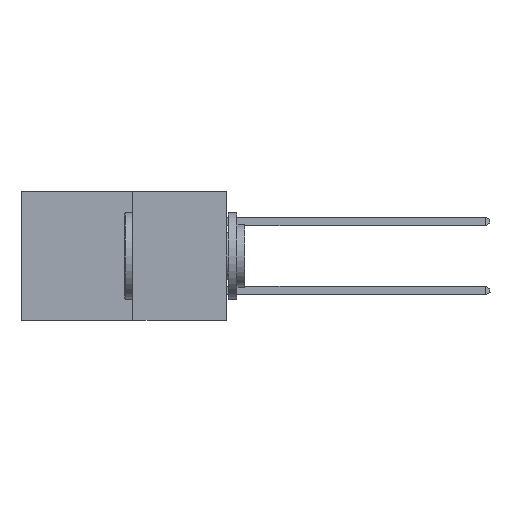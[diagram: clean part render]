
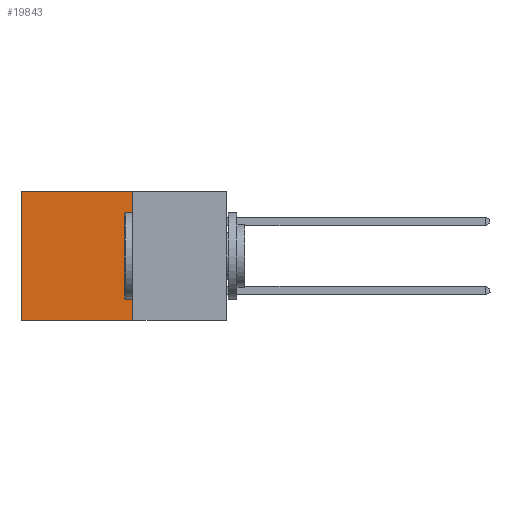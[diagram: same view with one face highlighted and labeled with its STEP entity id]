
A CAD part, left-side view. The second image highlights one B-rep face of the part: STEP entity #19843.
In plain terms, the highlighted planar face has unit normal (-1, 0, 0).
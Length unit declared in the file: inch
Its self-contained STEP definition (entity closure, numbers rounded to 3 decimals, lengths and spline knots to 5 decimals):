
#529 = EDGE_CURVE ( 'NONE', #17937, #8803, #17477, .T. ) ;
#590 = EDGE_CURVE ( 'NONE', #17795, #11460, #8284, .T. ) ;
#1274 = CARTESIAN_POINT ( 'NONE',  ( 0.277, 0.27, -0.37 ) ) ;
#2105 = CARTESIAN_POINT ( 'NONE',  ( 0.277, 0.27, 0. ) ) ;
#2142 = ORIENTED_EDGE ( 'NONE', *, *, #19636, .F. ) ;
#2510 = DIRECTION ( 'NONE',  ( 0., 0., -1. ) ) ;
#3514 = CARTESIAN_POINT ( 'NONE',  ( 0.277, 0.59, -0.37 ) ) ;
#4273 = EDGE_LOOP ( 'NONE', ( #13046, #2142, #16740, #10080 ) ) ;
#4469 = VECTOR ( 'NONE', #13166, 39.37008 ) ;
#4777 = CARTESIAN_POINT ( 'NONE',  ( 0.277, 0.59, -0.37 ) ) ;
#4942 = PLANE ( 'NONE',  #17885 ) ;
#6446 = CARTESIAN_POINT ( 'NONE',  ( 0.277, 0.27, 0. ) ) ;
#6563 = DIRECTION ( 'NONE',  ( 1., 0., 0. ) ) ;
#6834 = LINE ( 'NONE', #2105, #18254 ) ;
#7881 = LINE ( 'NONE', #1274, #12066 ) ;
#8284 = LINE ( 'NONE', #13213, #4469 ) ;
#8803 = VERTEX_POINT ( 'NONE', #4777 ) ;
#10080 = ORIENTED_EDGE ( 'NONE', *, *, #17344, .T. ) ;
#11460 = VERTEX_POINT ( 'NONE', #13291 ) ;
#11755 = DIRECTION ( 'NONE',  ( 0., 1., 0. ) ) ;
#12066 = VECTOR ( 'NONE', #12418, 39.37008 ) ;
#12418 = DIRECTION ( 'NONE',  ( 0., 1., 0. ) ) ;
#13046 = ORIENTED_EDGE ( 'NONE', *, *, #529, .T. ) ;
#13166 = DIRECTION ( 'NONE',  ( 0., 0., -1. ) ) ;
#13213 = CARTESIAN_POINT ( 'NONE',  ( 0.277, 0.27, -0.37 ) ) ;
#13291 = CARTESIAN_POINT ( 'NONE',  ( 0.277, 0.27, -0.37 ) ) ;
#13460 = VECTOR ( 'NONE', #2510, 39.37008 ) ;
#14470 = CARTESIAN_POINT ( 'NONE',  ( 0.277, 0.27, -0.37 ) ) ;
#15915 = FACE_OUTER_BOUND ( 'NONE', #4273, .T. ) ;
#16740 = ORIENTED_EDGE ( 'NONE', *, *, #590, .F. ) ;
#17344 = EDGE_CURVE ( 'NONE', #17795, #17937, #6834, .T. ) ;
#17476 = DIRECTION ( 'NONE',  ( 0., 0., -1. ) ) ;
#17477 = LINE ( 'NONE', #3514, #13460 ) ;
#17795 = VERTEX_POINT ( 'NONE', #6446 ) ;
#17885 = AXIS2_PLACEMENT_3D ( 'NONE', #14470, #6563, #17476 ) ;
#17937 = VERTEX_POINT ( 'NONE', #19119 ) ;
#18254 = VECTOR ( 'NONE', #11755, 39.37008 ) ;
#19119 = CARTESIAN_POINT ( 'NONE',  ( 0.277, 0.59, 0. ) ) ;
#19636 = EDGE_CURVE ( 'NONE', #11460, #8803, #7881, .T. ) ;
#19843 = ADVANCED_FACE ( 'NONE', ( #15915 ), #4942, .F. ) ;
